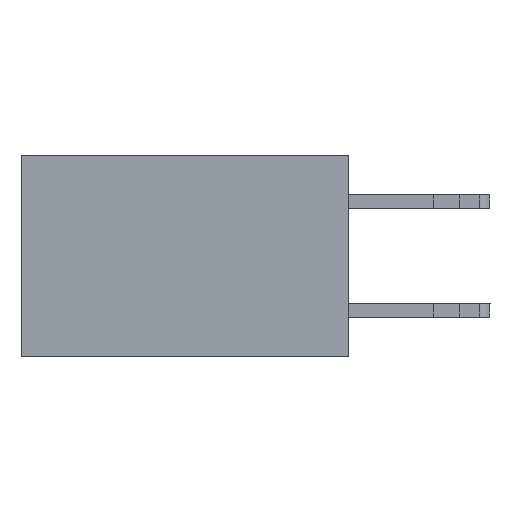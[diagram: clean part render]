
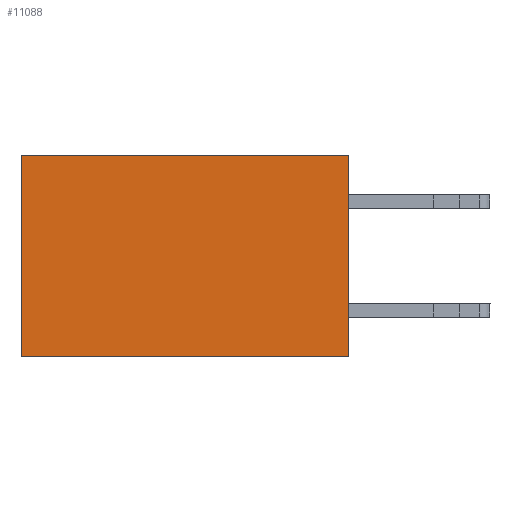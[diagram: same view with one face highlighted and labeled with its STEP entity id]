
A CAD part, left-side view. The second image highlights one B-rep face of the part: STEP entity #11088.
In plain terms, the highlighted planar face has unit normal (-1, 0, 0).
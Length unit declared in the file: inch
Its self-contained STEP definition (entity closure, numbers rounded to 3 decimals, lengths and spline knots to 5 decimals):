
#219 = LINE ( 'NONE', #12233, #17167 ) ;
#1974 = FACE_OUTER_BOUND ( 'NONE', #8218, .T. ) ;
#2058 = DIRECTION ( 'NONE',  ( 0., 0., -1. ) ) ;
#3525 = CARTESIAN_POINT ( 'NONE',  ( 0.2615, 0., -0.37 ) ) ;
#3808 = VECTOR ( 'NONE', #20374, 39.37008 ) ;
#4315 = ORIENTED_EDGE ( 'NONE', *, *, #15816, .T. ) ;
#4557 = DIRECTION ( 'NONE',  ( 0., 0., -1. ) ) ;
#6185 = EDGE_CURVE ( 'NONE', #6498, #9515, #219, .T. ) ;
#6197 = VECTOR ( 'NONE', #4557, 39.37008 ) ;
#6388 = CARTESIAN_POINT ( 'NONE',  ( 0.2615, 0.6, 0. ) ) ;
#6498 = VERTEX_POINT ( 'NONE', #6388 ) ;
#7010 = CARTESIAN_POINT ( 'NONE',  ( 0.2615, 0.6, -0.37 ) ) ;
#8218 = EDGE_LOOP ( 'NONE', ( #18618, #11925, #19897, #4315 ) ) ;
#9515 = VERTEX_POINT ( 'NONE', #7010 ) ;
#10339 = CARTESIAN_POINT ( 'NONE',  ( 0.2615, 0., -0.37 ) ) ;
#11088 = ADVANCED_FACE ( 'NONE', ( #1974 ), #19831, .F. ) ;
#11925 = ORIENTED_EDGE ( 'NONE', *, *, #13273, .F. ) ;
#11949 = DIRECTION ( 'NONE',  ( 1., 0., 0. ) ) ;
#11988 = DIRECTION ( 'NONE',  ( 0., 0., -1. ) ) ;
#12136 = CARTESIAN_POINT ( 'NONE',  ( 0.2615, 0., 0. ) ) ;
#12233 = CARTESIAN_POINT ( 'NONE',  ( 0.2615, 0.6, -0.37 ) ) ;
#13244 = LINE ( 'NONE', #14237, #6197 ) ;
#13273 = EDGE_CURVE ( 'NONE', #20665, #9515, #20847, .T. ) ;
#13877 = AXIS2_PLACEMENT_3D ( 'NONE', #10339, #11949, #2058 ) ;
#14237 = CARTESIAN_POINT ( 'NONE',  ( 0.2615, 0., -0.37 ) ) ;
#15105 = LINE ( 'NONE', #12136, #18806 ) ;
#15344 = DIRECTION ( 'NONE',  ( 0., 1., 0. ) ) ;
#15632 = CARTESIAN_POINT ( 'NONE',  ( 0.2615, 0., -0.37 ) ) ;
#15816 = EDGE_CURVE ( 'NONE', #20844, #6498, #15105, .T. ) ;
#16867 = CARTESIAN_POINT ( 'NONE',  ( 0.2615, 0., 0. ) ) ;
#17167 = VECTOR ( 'NONE', #11988, 39.37008 ) ;
#18314 = EDGE_CURVE ( 'NONE', #20844, #20665, #13244, .T. ) ;
#18618 = ORIENTED_EDGE ( 'NONE', *, *, #6185, .T. ) ;
#18806 = VECTOR ( 'NONE', #15344, 39.37008 ) ;
#19831 = PLANE ( 'NONE',  #13877 ) ;
#19897 = ORIENTED_EDGE ( 'NONE', *, *, #18314, .F. ) ;
#20374 = DIRECTION ( 'NONE',  ( 0., 1., 0. ) ) ;
#20665 = VERTEX_POINT ( 'NONE', #3525 ) ;
#20844 = VERTEX_POINT ( 'NONE', #16867 ) ;
#20847 = LINE ( 'NONE', #15632, #3808 ) ;
